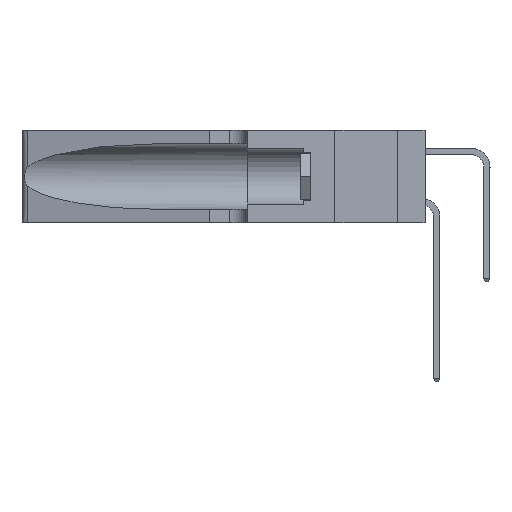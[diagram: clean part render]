
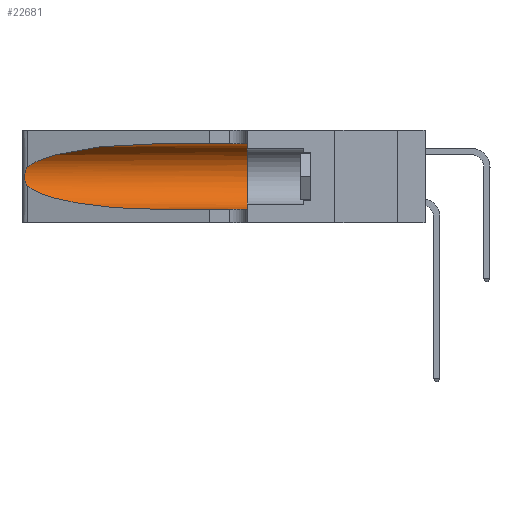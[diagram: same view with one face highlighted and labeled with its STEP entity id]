
A CAD part, left-side view. The second image highlights one B-rep face of the part: STEP entity #22681.
In plain terms, the highlighted cylindrical face has radius 3.308 mm (diameter 6.617 mm), a partial arc.
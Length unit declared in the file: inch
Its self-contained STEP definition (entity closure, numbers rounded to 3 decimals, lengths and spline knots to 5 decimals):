
#918 = CARTESIAN_POINT ( 'NONE',  ( 0.25639, 1.23184, 0.21858 ) ) ;
#971 = DIRECTION ( 'NONE',  ( 0., -1., 0. ) ) ;
#1076 = CARTESIAN_POINT ( 'NONE',  ( 0.25555, 1.22993, 0.14849 ) ) ;
#1480 = ORIENTED_EDGE ( 'NONE', *, *, #36830, .T. ) ;
#3236 = DIRECTION ( 'NONE',  ( 0., -1., 0. ) ) ;
#4594 = CARTESIAN_POINT ( 'NONE',  ( 0.25487, 1.22718, 0.22369 ) ) ;
#6002 = CARTESIAN_POINT ( 'NONE',  ( 0.1305, 0.35, 0.05475 ) ) ;
#6090 = FACE_OUTER_BOUND ( 'NONE', #37166, .T. ) ;
#7615 = VERTEX_POINT ( 'NONE', #6002 ) ;
#7964 = EDGE_CURVE ( 'NONE', #40105, #7615, #36550, .T. ) ;
#8259 = CARTESIAN_POINT ( 'NONE',  ( 0.25787, 1.23484, 0.2124 ) ) ;
#8749 = CARTESIAN_POINT ( 'NONE',  ( 0.1305, 0.72297, 0.31525 ) ) ;
#9223 = EDGE_CURVE ( 'NONE', #38266, #37279, #44141, .T. ) ;
#9598 = VECTOR ( 'NONE', #971, 39.37008 ) ;
#10107 = CARTESIAN_POINT ( 'NONE',  ( 0.25487, 1.22718, 0.22369 ) ) ;
#11497 = DIRECTION ( 'NONE',  ( 0., 1., 0. ) ) ;
#11871 = ORIENTED_EDGE ( 'NONE', *, *, #7964, .F. ) ;
#11885 = CARTESIAN_POINT ( 'NONE',  ( 0.26018, 1.23835, 0.19895 ) ) ;
#11927 = DIRECTION ( 'NONE',  ( 0., 0., -1. ) ) ;
#12801 = VECTOR ( 'NONE', #3236, 39.37008 ) ;
#13097 = EDGE_CURVE ( 'NONE', #18716, #38266, #27531, .T. ) ;
#15546 = CARTESIAN_POINT ( 'NONE',  ( 0.26075, 1.23896, 0.178 ) ) ;
#15699 =( BOUNDED_CURVE ( )  B_SPLINE_CURVE ( 3, ( #28538, #32179, #17832, #42919 ),
 .UNSPECIFIED., .F., .F. ) 
 B_SPLINE_CURVE_WITH_KNOTS ( ( 4, 4 ),
 ( 3.44316, 4.71239 ),
 .UNSPECIFIED. ) 
 CURVE ( )  GEOMETRIC_REPRESENTATION_ITEM ( )  RATIONAL_B_SPLINE_CURVE ( ( 1., 0.87, 0.87, 1. ) ) 
 REPRESENTATION_ITEM ( '' )  );
#16867 = CARTESIAN_POINT ( 'NONE',  ( 0.1305, 0.72297, 0.31525 ) ) ;
#17832 = CARTESIAN_POINT ( 'NONE',  ( 0.18966, 0.96281, 0.05475 ) ) ;
#18716 = VERTEX_POINT ( 'NONE', #16867 ) ;
#19173 = CARTESIAN_POINT ( 'NONE',  ( 0.25856, 1.23593, 0.16098 ) ) ;
#19681 = CARTESIAN_POINT ( 'NONE',  ( 0.25487, 1.22718, 0.22369 ) ) ;
#21818 = VERTEX_POINT ( 'NONE', #44799 ) ;
#22681 = ADVANCED_FACE ( 'NONE', ( #6090 ), #33740, .F. ) ;
#22751 = CARTESIAN_POINT ( 'NONE',  ( 0.1305, 1.61858, 0.31525 ) ) ;
#22851 = CARTESIAN_POINT ( 'NONE',  ( 0.25639, 1.23186, 0.15144 ) ) ;
#23026 = ORIENTED_EDGE ( 'NONE', *, *, #9223, .T. ) ;
#23393 = EDGE_CURVE ( 'NONE', #21818, #7615, #41489, .T. ) ;
#24727 = CARTESIAN_POINT ( 'NONE',  ( 0.1305, 0.35, 0.31525 ) ) ;
#26272 = CARTESIAN_POINT ( 'NONE',  ( 0.25555, 1.22994, 0.2215 ) ) ;
#26435 = CARTESIAN_POINT ( 'NONE',  ( 0.25487, 1.22718, 0.14631 ) ) ;
#27531 =( BOUNDED_CURVE ( )  B_SPLINE_CURVE ( 3, ( #8749, #37588, #41161, #19681 ),
 .UNSPECIFIED., .F., .F. ) 
 B_SPLINE_CURVE_WITH_KNOTS ( ( 4, 4 ),
 ( 1.5708, 2.84003 ),
 .UNSPECIFIED. ) 
 CURVE ( )  GEOMETRIC_REPRESENTATION_ITEM ( )  RATIONAL_B_SPLINE_CURVE ( ( 1., 0.87, 0.87, 1. ) ) 
 REPRESENTATION_ITEM ( '' )  );
#27965 = EDGE_CURVE ( 'NONE', #18716, #40105, #45597, .T. ) ;
#28538 = CARTESIAN_POINT ( 'NONE',  ( 0.25487, 1.22718, 0.14631 ) ) ;
#29918 = DIRECTION ( 'NONE',  ( 0., -1., 0. ) ) ;
#30279 = ORIENTED_EDGE ( 'NONE', *, *, #27965, .F. ) ;
#31032 = CARTESIAN_POINT ( 'NONE',  ( 0.25487, 1.22718, 0.14631 ) ) ;
#32179 = CARTESIAN_POINT ( 'NONE',  ( 0.2373, 1.15595, 0.08982 ) ) ;
#32902 = ORIENTED_EDGE ( 'NONE', *, *, #23393, .T. ) ;
#33120 = CARTESIAN_POINT ( 'NONE',  ( 0.1305, 0.35, 0.185 ) ) ;
#33487 = CARTESIAN_POINT ( 'NONE',  ( 0.25854, 1.2359, 0.20912 ) ) ;
#33523 = CARTESIAN_POINT ( 'NONE',  ( 0.1305, 1.61858, 0.185 ) ) ;
#33740 = CYLINDRICAL_SURFACE ( 'NONE', #40554, 0.13025 ) ;
#34755 = AXIS2_PLACEMENT_3D ( 'NONE', #33120, #11497, #36712 ) ;
#36550 = CIRCLE ( 'NONE', #34755, 0.13025 ) ;
#36712 = DIRECTION ( 'NONE',  ( 0., 0., 1. ) ) ;
#36830 = EDGE_CURVE ( 'NONE', #37279, #21818, #15699, .T. ) ;
#37080 = CARTESIAN_POINT ( 'NONE',  ( 0.26075, 1.23896, 0.19203 ) ) ;
#37166 = EDGE_LOOP ( 'NONE', ( #45018, #23026, #1480, #32902, #11871, #30279 ) ) ;
#37279 = VERTEX_POINT ( 'NONE', #31032 ) ;
#37588 = CARTESIAN_POINT ( 'NONE',  ( 0.18966, 0.96281, 0.31525 ) ) ;
#38266 = VERTEX_POINT ( 'NONE', #10107 ) ;
#40105 = VERTEX_POINT ( 'NONE', #24727 ) ;
#40554 = AXIS2_PLACEMENT_3D ( 'NONE', #33523, #29918, #11927 ) ;
#40674 = CARTESIAN_POINT ( 'NONE',  ( 0.26017, 1.23833, 0.17102 ) ) ;
#41161 = CARTESIAN_POINT ( 'NONE',  ( 0.2373, 1.15595, 0.28018 ) ) ;
#41489 = LINE ( 'NONE', #46358, #12801 ) ;
#42919 = CARTESIAN_POINT ( 'NONE',  ( 0.1305, 0.72297, 0.05475 ) ) ;
#44141 = B_SPLINE_CURVE_WITH_KNOTS ( 'NONE', 3,
 ( #4594, #26272, #918, #8259, #33487, #11885, #37080, #15546, #40674, #19173, #44230, #22851, #1076, #26435 ),
 .UNSPECIFIED., .F., .F.,
 ( 4, 2, 2, 2, 2, 2, 4 ),
 ( 0., 0.00027, 0.00053, 0.00107, 0.0016, 0.00187, 0.00214 ),
 .UNSPECIFIED. ) ;
#44230 = CARTESIAN_POINT ( 'NONE',  ( 0.25789, 1.23486, 0.15765 ) ) ;
#44799 = CARTESIAN_POINT ( 'NONE',  ( 0.1305, 0.72297, 0.05475 ) ) ;
#45018 = ORIENTED_EDGE ( 'NONE', *, *, #13097, .T. ) ;
#45597 = LINE ( 'NONE', #22751, #9598 ) ;
#46358 = CARTESIAN_POINT ( 'NONE',  ( 0.1305, 1.61858, 0.05475 ) ) ;
